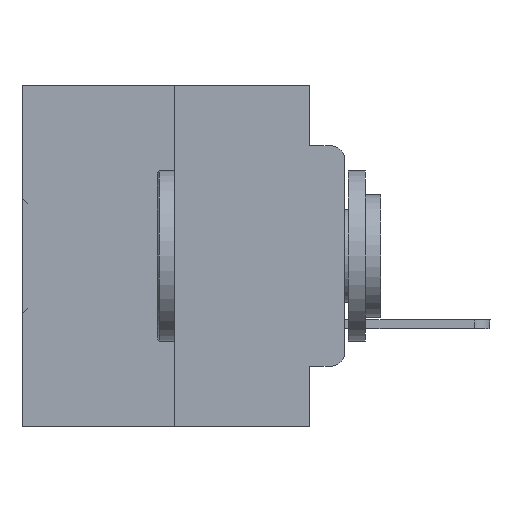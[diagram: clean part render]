
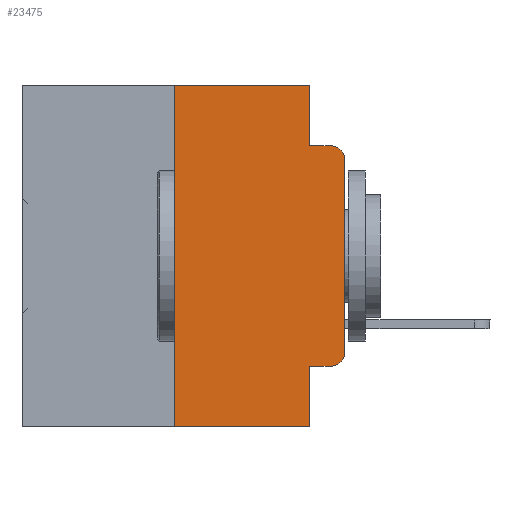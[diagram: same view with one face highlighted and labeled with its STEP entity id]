
A CAD part, left-side view. The second image highlights one B-rep face of the part: STEP entity #23475.
In plain terms, the highlighted planar face has unit normal (-1, 0, 0).
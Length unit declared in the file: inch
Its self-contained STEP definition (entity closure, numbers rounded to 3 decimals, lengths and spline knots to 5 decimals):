
#464 = EDGE_CURVE ( 'NONE', #11492, #10814, #28322, .T. ) ;
#512 = VERTEX_POINT ( 'NONE', #6444 ) ;
#519 = EDGE_CURVE ( 'NONE', #11528, #33243, #30876, .T. ) ;
#902 = LINE ( 'NONE', #10913, #16476 ) ;
#1127 = CARTESIAN_POINT ( 'NONE',  ( 0., 0.051, -0.4115 ) ) ;
#1234 = LINE ( 'NONE', #23947, #14133 ) ;
#1398 = VERTEX_POINT ( 'NONE', #5485 ) ;
#1584 = VECTOR ( 'NONE', #23553, 39.37008 ) ;
#1966 = CARTESIAN_POINT ( 'NONE',  ( 0., 0.02, -0.3915 ) ) ;
#3446 = ORIENTED_EDGE ( 'NONE', *, *, #5682, .T. ) ;
#3833 = DIRECTION ( 'NONE',  ( 0., -1., 0. ) ) ;
#4422 = CARTESIAN_POINT ( 'NONE',  ( 0., 0.051, 0. ) ) ;
#4620 = LINE ( 'NONE', #25686, #19229 ) ;
#4768 = ORIENTED_EDGE ( 'NONE', *, *, #16916, .T. ) ;
#5076 = LINE ( 'NONE', #23800, #1584 ) ;
#5456 = CARTESIAN_POINT ( 'NONE',  ( 0., 0.051, 0. ) ) ;
#5485 = CARTESIAN_POINT ( 'NONE',  ( 0., 0.02, -0.0885 ) ) ;
#5682 = EDGE_CURVE ( 'NONE', #11528, #7396, #31949, .T. ) ;
#5832 = EDGE_CURVE ( 'NONE', #28013, #30234, #902, .T. ) ;
#6444 = CARTESIAN_POINT ( 'NONE',  ( 0., 0., -0.1085 ) ) ;
#7396 = VERTEX_POINT ( 'NONE', #33412 ) ;
#8228 = AXIS2_PLACEMENT_3D ( 'NONE', #23043, #23282, #9223 ) ;
#8547 = ORIENTED_EDGE ( 'NONE', *, *, #5832, .F. ) ;
#8748 = ORIENTED_EDGE ( 'NONE', *, *, #519, .F. ) ;
#9151 = VECTOR ( 'NONE', #3833, 39.37008 ) ;
#9223 = DIRECTION ( 'NONE',  ( 0., 0., -1. ) ) ;
#9486 = DIRECTION ( 'NONE',  ( 0., -1., 0. ) ) ;
#9629 = FACE_OUTER_BOUND ( 'NONE', #25213, .T. ) ;
#10814 = VERTEX_POINT ( 'NONE', #14748 ) ;
#10912 = CARTESIAN_POINT ( 'NONE',  ( 0., 0.051, -0.5 ) ) ;
#10913 = CARTESIAN_POINT ( 'NONE',  ( 0., 0.25, 0. ) ) ;
#11023 = DIRECTION ( 'NONE',  ( 0., 0., 1. ) ) ;
#11492 = VERTEX_POINT ( 'NONE', #4422 ) ;
#11528 = VERTEX_POINT ( 'NONE', #1127 ) ;
#13128 = EDGE_CURVE ( 'NONE', #7396, #14480, #31156, .T. ) ;
#13702 = ORIENTED_EDGE ( 'NONE', *, *, #13128, .T. ) ;
#13737 = DIRECTION ( 'NONE',  ( 0., 0., -1. ) ) ;
#13873 = CARTESIAN_POINT ( 'NONE',  ( 0., 0.25, 0. ) ) ;
#14090 = CARTESIAN_POINT ( 'NONE',  ( 0., 0.25, -0.5 ) ) ;
#14133 = VECTOR ( 'NONE', #32807, 39.37008 ) ;
#14480 = VERTEX_POINT ( 'NONE', #34696 ) ;
#14748 = CARTESIAN_POINT ( 'NONE',  ( 0., 0.051, -0.0885 ) ) ;
#14992 = PLANE ( 'NONE',  #8228 ) ;
#15498 = LINE ( 'NONE', #16392, #30462 ) ;
#16000 = CIRCLE ( 'NONE', #33677, 0.02 ) ;
#16392 = CARTESIAN_POINT ( 'NONE',  ( 0., 0.473, -0.5 ) ) ;
#16476 = VECTOR ( 'NONE', #11023, 39.37008 ) ;
#16916 = EDGE_CURVE ( 'NONE', #14480, #512, #1234, .T. ) ;
#17468 = ORIENTED_EDGE ( 'NONE', *, *, #21908, .F. ) ;
#18487 = VECTOR ( 'NONE', #31405, 39.37008 ) ;
#19068 = ORIENTED_EDGE ( 'NONE', *, *, #464, .F. ) ;
#19229 = VECTOR ( 'NONE', #9486, 39.37008 ) ;
#19486 = CARTESIAN_POINT ( 'NONE',  ( 0., 0.02, -0.1085 ) ) ;
#19828 = DIRECTION ( 'NONE',  ( 0., 0., -1. ) ) ;
#20303 = CARTESIAN_POINT ( 'NONE',  ( 0., 0.051, -0.4115 ) ) ;
#21118 = EDGE_CURVE ( 'NONE', #30234, #11492, #5076, .T. ) ;
#21908 = EDGE_CURVE ( 'NONE', #10814, #1398, #4620, .T. ) ;
#23043 = CARTESIAN_POINT ( 'NONE',  ( 0., 0.473, 0. ) ) ;
#23282 = DIRECTION ( 'NONE',  ( 1., 0., 0. ) ) ;
#23475 = ADVANCED_FACE ( 'NONE', ( #9629 ), #14992, .F. ) ;
#23553 = DIRECTION ( 'NONE',  ( 0., -1., 0. ) ) ;
#23800 = CARTESIAN_POINT ( 'NONE',  ( 0., 0.473, 0. ) ) ;
#23947 = CARTESIAN_POINT ( 'NONE',  ( 0., 0., 0. ) ) ;
#25213 = EDGE_LOOP ( 'NONE', ( #4768, #28436, #17468, #19068, #33119, #8547, #25666, #8748, #3446, #13702 ) ) ;
#25666 = ORIENTED_EDGE ( 'NONE', *, *, #30997, .T. ) ;
#25686 = CARTESIAN_POINT ( 'NONE',  ( 0., 0.051, -0.0885 ) ) ;
#27521 = AXIS2_PLACEMENT_3D ( 'NONE', #1966, #29226, #31844 ) ;
#28013 = VERTEX_POINT ( 'NONE', #14090 ) ;
#28322 = LINE ( 'NONE', #5456, #31766 ) ;
#28436 = ORIENTED_EDGE ( 'NONE', *, *, #30430, .T. ) ;
#28767 = CARTESIAN_POINT ( 'NONE',  ( 0., 0.051, 0. ) ) ;
#29226 = DIRECTION ( 'NONE',  ( -1., 0., 0. ) ) ;
#30171 = DIRECTION ( 'NONE',  ( 0., -1., 0. ) ) ;
#30234 = VERTEX_POINT ( 'NONE', #13873 ) ;
#30430 = EDGE_CURVE ( 'NONE', #512, #1398, #16000, .T. ) ;
#30462 = VECTOR ( 'NONE', #30171, 39.37008 ) ;
#30876 = LINE ( 'NONE', #28767, #18487 ) ;
#30997 = EDGE_CURVE ( 'NONE', #28013, #33243, #15498, .T. ) ;
#31156 = CIRCLE ( 'NONE', #27521, 0.02 ) ;
#31405 = DIRECTION ( 'NONE',  ( 0., 0., -1. ) ) ;
#31766 = VECTOR ( 'NONE', #13737, 39.37008 ) ;
#31844 = DIRECTION ( 'NONE',  ( 0., 0., -1. ) ) ;
#31949 = LINE ( 'NONE', #20303, #9151 ) ;
#32807 = DIRECTION ( 'NONE',  ( 0., 0., 1. ) ) ;
#33119 = ORIENTED_EDGE ( 'NONE', *, *, #21118, .F. ) ;
#33243 = VERTEX_POINT ( 'NONE', #10912 ) ;
#33395 = DIRECTION ( 'NONE',  ( -1., 0., 0. ) ) ;
#33412 = CARTESIAN_POINT ( 'NONE',  ( 0., 0.02, -0.4115 ) ) ;
#33677 = AXIS2_PLACEMENT_3D ( 'NONE', #19486, #33395, #19828 ) ;
#34696 = CARTESIAN_POINT ( 'NONE',  ( 0., 0., -0.3915 ) ) ;
